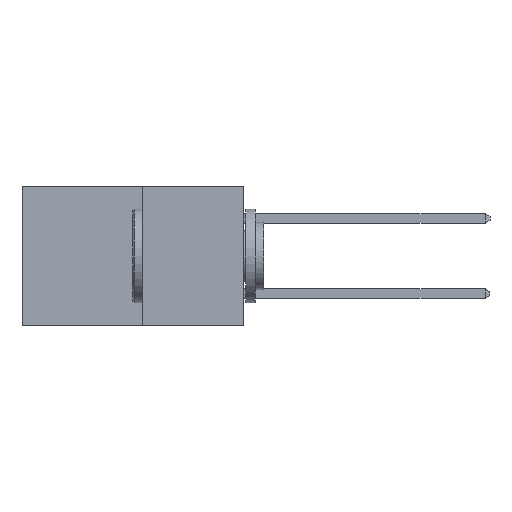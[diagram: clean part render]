
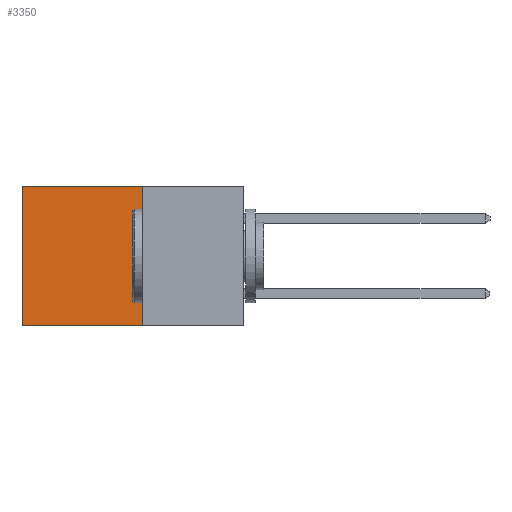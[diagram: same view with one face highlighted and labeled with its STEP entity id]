
A CAD part, left-side view. The second image highlights one B-rep face of the part: STEP entity #3350.
In plain terms, the highlighted planar face has unit normal (-1, 0, 0).
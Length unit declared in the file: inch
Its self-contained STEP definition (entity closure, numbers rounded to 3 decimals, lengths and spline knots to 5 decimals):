
#790 = VECTOR ( 'NONE', #4788, 39.37008 ) ;
#1085 = VERTEX_POINT ( 'NONE', #3571 ) ;
#1107 = DIRECTION ( 'NONE',  ( 0., 1., 0. ) ) ;
#1676 = EDGE_CURVE ( 'NONE', #1085, #6997, #2539, .T. ) ;
#1730 = VECTOR ( 'NONE', #1107, 39.37008 ) ;
#1938 = VERTEX_POINT ( 'NONE', #6103 ) ;
#2103 = VECTOR ( 'NONE', #4514, 39.37008 ) ;
#2350 = EDGE_CURVE ( 'NONE', #4892, #1938, #6467, .T. ) ;
#2352 = VECTOR ( 'NONE', #5267, 39.37008 ) ;
#2438 = EDGE_CURVE ( 'NONE', #6997, #1938, #2651, .T. ) ;
#2539 = LINE ( 'NONE', #5565, #2352 ) ;
#2618 = CARTESIAN_POINT ( 'NONE',  ( 0.277, 0.27, -0.37 ) ) ;
#2651 = LINE ( 'NONE', #4862, #790 ) ;
#2791 = AXIS2_PLACEMENT_3D ( 'NONE', #7640, #7613, #7595 ) ;
#2935 = CARTESIAN_POINT ( 'NONE',  ( 0.277, 0.27, -0.37 ) ) ;
#3350 = ADVANCED_FACE ( 'NONE', ( #4342 ), #7677, .F. ) ;
#3571 = CARTESIAN_POINT ( 'NONE',  ( 0.277, 0.27, 0. ) ) ;
#3834 = LINE ( 'NONE', #3921, #2103 ) ;
#3921 = CARTESIAN_POINT ( 'NONE',  ( 0.277, 0.27, -0.37 ) ) ;
#3946 = CARTESIAN_POINT ( 'NONE',  ( 0.277, 0.59, 0. ) ) ;
#4342 = FACE_OUTER_BOUND ( 'NONE', #5113, .T. ) ;
#4443 = ORIENTED_EDGE ( 'NONE', *, *, #2350, .F. ) ;
#4514 = DIRECTION ( 'NONE',  ( 0., 0., -1. ) ) ;
#4655 = ORIENTED_EDGE ( 'NONE', *, *, #1676, .T. ) ;
#4788 = DIRECTION ( 'NONE',  ( 0., 0., -1. ) ) ;
#4862 = CARTESIAN_POINT ( 'NONE',  ( 0.277, 0.59, -0.37 ) ) ;
#4892 = VERTEX_POINT ( 'NONE', #2935 ) ;
#5113 = EDGE_LOOP ( 'NONE', ( #5956, #4443, #6160, #4655 ) ) ;
#5267 = DIRECTION ( 'NONE',  ( 0., 1., 0. ) ) ;
#5565 = CARTESIAN_POINT ( 'NONE',  ( 0.277, 0.27, 0. ) ) ;
#5956 = ORIENTED_EDGE ( 'NONE', *, *, #2438, .T. ) ;
#6103 = CARTESIAN_POINT ( 'NONE',  ( 0.277, 0.59, -0.37 ) ) ;
#6160 = ORIENTED_EDGE ( 'NONE', *, *, #8285, .F. ) ;
#6467 = LINE ( 'NONE', #2618, #1730 ) ;
#6997 = VERTEX_POINT ( 'NONE', #3946 ) ;
#7595 = DIRECTION ( 'NONE',  ( 0., 0., -1. ) ) ;
#7613 = DIRECTION ( 'NONE',  ( 1., 0., 0. ) ) ;
#7640 = CARTESIAN_POINT ( 'NONE',  ( 0.277, 0.27, -0.37 ) ) ;
#7677 = PLANE ( 'NONE',  #2791 ) ;
#8285 = EDGE_CURVE ( 'NONE', #1085, #4892, #3834, .T. ) ;
